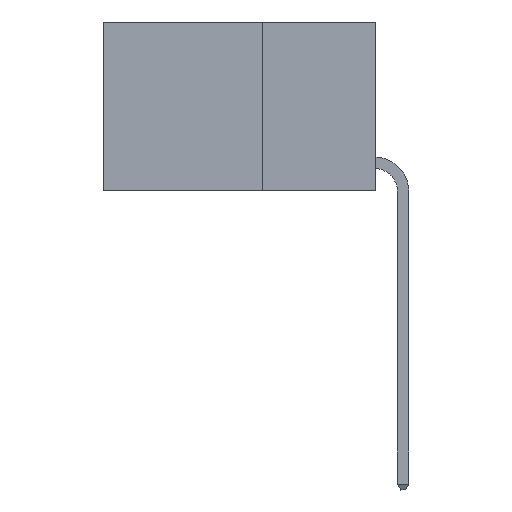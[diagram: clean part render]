
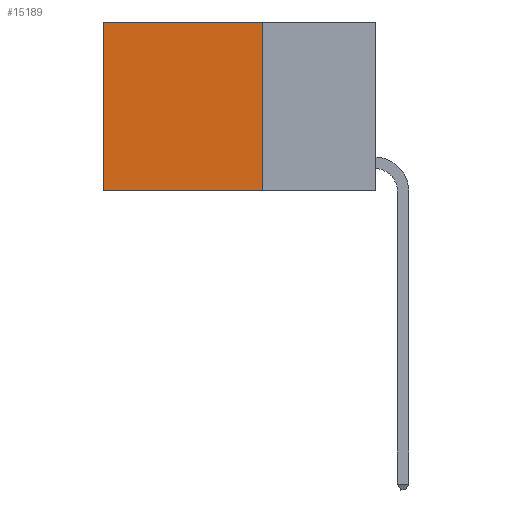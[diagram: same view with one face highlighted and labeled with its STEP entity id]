
A CAD part, left-side view. The second image highlights one B-rep face of the part: STEP entity #15189.
In plain terms, the highlighted planar face has unit normal (-1, 0, 0).
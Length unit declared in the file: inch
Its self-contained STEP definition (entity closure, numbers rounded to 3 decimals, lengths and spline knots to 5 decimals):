
#614 = CARTESIAN_POINT ( 'NONE',  ( 0.2625, 0.25, 0. ) ) ;
#2271 = ORIENTED_EDGE ( 'NONE', *, *, #13302, .F. ) ;
#2286 = EDGE_LOOP ( 'NONE', ( #20809, #2271, #13532, #10357 ) ) ;
#2371 = VECTOR ( 'NONE', #8594, 39.37008 ) ;
#2387 = DIRECTION ( 'NONE',  ( 1., 0., 0. ) ) ;
#2923 = VERTEX_POINT ( 'NONE', #22340 ) ;
#3205 = DIRECTION ( 'NONE',  ( 0., 1., 0. ) ) ;
#4606 = CARTESIAN_POINT ( 'NONE',  ( 0.2625, 0.6, 0. ) ) ;
#4965 = CARTESIAN_POINT ( 'NONE',  ( 0.2625, 0.25, -0.37 ) ) ;
#5553 = LINE ( 'NONE', #14585, #14264 ) ;
#5912 = DIRECTION ( 'NONE',  ( 0., 1., 0. ) ) ;
#6609 = VECTOR ( 'NONE', #10398, 39.37008 ) ;
#6779 = VERTEX_POINT ( 'NONE', #20923 ) ;
#6997 = LINE ( 'NONE', #10260, #2371 ) ;
#7068 = VERTEX_POINT ( 'NONE', #18248 ) ;
#7241 = VECTOR ( 'NONE', #3205, 39.37008 ) ;
#8340 = LINE ( 'NONE', #4965, #7241 ) ;
#8594 = DIRECTION ( 'NONE',  ( 0., 0., -1. ) ) ;
#10260 = CARTESIAN_POINT ( 'NONE',  ( 0.2625, 0.6, 0. ) ) ;
#10357 = ORIENTED_EDGE ( 'NONE', *, *, #14568, .T. ) ;
#10398 = DIRECTION ( 'NONE',  ( 0., 0., -1. ) ) ;
#11810 = LINE ( 'NONE', #13889, #6609 ) ;
#13302 = EDGE_CURVE ( 'NONE', #6779, #7068, #8340, .T. ) ;
#13318 = AXIS2_PLACEMENT_3D ( 'NONE', #614, #2387, #14558 ) ;
#13532 = ORIENTED_EDGE ( 'NONE', *, *, #14929, .F. ) ;
#13889 = CARTESIAN_POINT ( 'NONE',  ( 0.2625, 0.25, 0. ) ) ;
#14264 = VECTOR ( 'NONE', #5912, 39.37008 ) ;
#14558 = DIRECTION ( 'NONE',  ( 0., 0., -1. ) ) ;
#14568 = EDGE_CURVE ( 'NONE', #2923, #16802, #5553, .T. ) ;
#14585 = CARTESIAN_POINT ( 'NONE',  ( 0.2625, 0.25, 0. ) ) ;
#14929 = EDGE_CURVE ( 'NONE', #2923, #6779, #11810, .T. ) ;
#15189 = ADVANCED_FACE ( 'NONE', ( #15570 ), #21395, .F. ) ;
#15570 = FACE_OUTER_BOUND ( 'NONE', #2286, .T. ) ;
#16802 = VERTEX_POINT ( 'NONE', #4606 ) ;
#18248 = CARTESIAN_POINT ( 'NONE',  ( 0.2625, 0.6, -0.37 ) ) ;
#20809 = ORIENTED_EDGE ( 'NONE', *, *, #22281, .T. ) ;
#20923 = CARTESIAN_POINT ( 'NONE',  ( 0.2625, 0.25, -0.37 ) ) ;
#21395 = PLANE ( 'NONE',  #13318 ) ;
#22281 = EDGE_CURVE ( 'NONE', #16802, #7068, #6997, .T. ) ;
#22340 = CARTESIAN_POINT ( 'NONE',  ( 0.2625, 0.25, 0. ) ) ;
